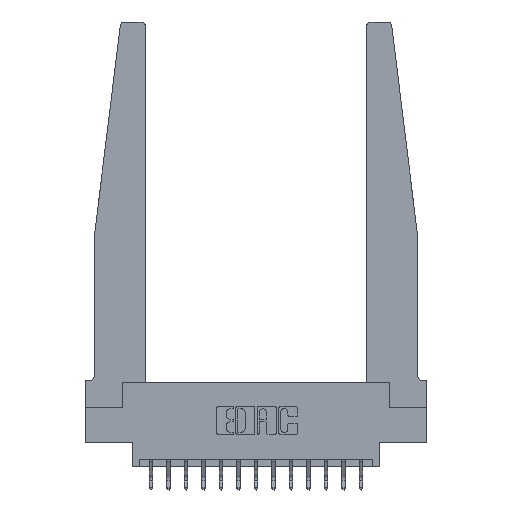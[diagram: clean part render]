
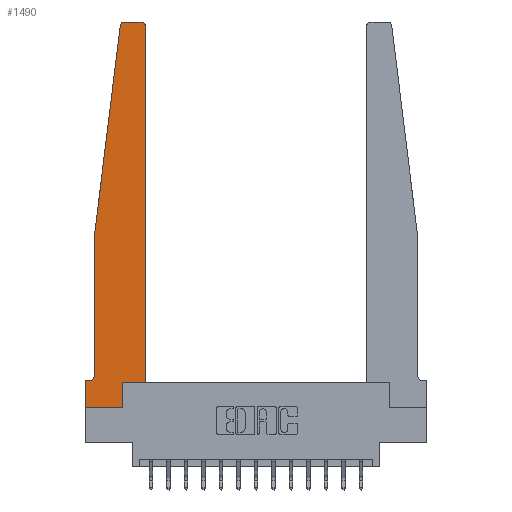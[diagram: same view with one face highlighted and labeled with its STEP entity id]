
A CAD part, top view. The second image highlights one B-rep face of the part: STEP entity #1490.
In plain terms, the highlighted planar face has unit normal (0, 0, 1).
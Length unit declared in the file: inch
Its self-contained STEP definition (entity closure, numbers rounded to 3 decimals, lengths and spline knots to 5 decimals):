
#187 = VECTOR ( 'NONE', #11471, 39.37008 ) ;
#728 = CARTESIAN_POINT ( 'NONE',  ( 0.25, 2.75, 0.37 ) ) ;
#776 = CARTESIAN_POINT ( 'NONE',  ( 0., 0., 0.37 ) ) ;
#872 = VERTEX_POINT ( 'NONE', #11358 ) ;
#966 = ORIENTED_EDGE ( 'NONE', *, *, #14735, .T. ) ;
#1274 = CARTESIAN_POINT ( 'NONE',  ( 0.065, 1.25, 0.37 ) ) ;
#1490 = ADVANCED_FACE ( 'NONE', ( #2339 ), #7859, .T. ) ;
#1570 = EDGE_CURVE ( 'NONE', #10822, #872, #14530, .T. ) ;
#1797 = DIRECTION ( 'NONE',  ( 0., 1., 0. ) ) ;
#1819 = CARTESIAN_POINT ( 'NONE',  ( 0.015, 0.1875, 0.37 ) ) ;
#1842 = CARTESIAN_POINT ( 'NONE',  ( 0.065, 1.25, 0.37 ) ) ;
#2105 = DIRECTION ( 'NONE',  ( -1., 0., 0. ) ) ;
#2115 = CARTESIAN_POINT ( 'NONE',  ( 0.065, 0.1875, 0.37 ) ) ;
#2339 = FACE_OUTER_BOUND ( 'NONE', #6630, .T. ) ;
#2379 = VERTEX_POINT ( 'NONE', #7065 ) ;
#2647 = AXIS2_PLACEMENT_3D ( 'NONE', #6317, #8947, #15874 ) ;
#2870 = CARTESIAN_POINT ( 'NONE',  ( 0., 0., 0.37 ) ) ;
#3141 = CARTESIAN_POINT ( 'NONE',  ( 0., 0., 0.37 ) ) ;
#3381 = LINE ( 'NONE', #2115, #16720 ) ;
#3712 = EDGE_CURVE ( 'NONE', #8958, #10822, #7441, .T. ) ;
#3829 = DIRECTION ( 'NONE',  ( -1., 0., 0. ) ) ;
#3869 = CARTESIAN_POINT ( 'NONE',  ( 0.395, 2.75, 0.37 ) ) ;
#3873 = CARTESIAN_POINT ( 'NONE',  ( 0.425, 0.18, 0.37 ) ) ;
#3912 = EDGE_CURVE ( 'NONE', #17514, #8958, #4047, .T. ) ;
#4047 = CIRCLE ( 'NONE', #14783, 0.03 ) ;
#4103 = CARTESIAN_POINT ( 'NONE',  ( 0.015, 0.2375, 0.37 ) ) ;
#4135 = DIRECTION ( 'NONE',  ( 1., 0., 0. ) ) ;
#4212 = LINE ( 'NONE', #2870, #187 ) ;
#4487 = DIRECTION ( 'NONE',  ( 0., 0., 1. ) ) ;
#4674 = EDGE_CURVE ( 'NONE', #11817, #5518, #9313, .T. ) ;
#4804 = DIRECTION ( 'NONE',  ( 0., -1., 0. ) ) ;
#4832 = ORIENTED_EDGE ( 'NONE', *, *, #9189, .T. ) ;
#4980 = EDGE_CURVE ( 'NONE', #16429, #11817, #14541, .T. ) ;
#5044 = ORIENTED_EDGE ( 'NONE', *, *, #12420, .T. ) ;
#5389 = CARTESIAN_POINT ( 'NONE',  ( 0.27653, 2.72, 0.37 ) ) ;
#5518 = VERTEX_POINT ( 'NONE', #1819 ) ;
#5753 = LINE ( 'NONE', #3141, #9712 ) ;
#5866 = EDGE_CURVE ( 'NONE', #2379, #6545, #16108, .T. ) ;
#5944 = CARTESIAN_POINT ( 'NONE',  ( 0.2605, 0.18, 0.37 ) ) ;
#6261 = DIRECTION ( 'NONE',  ( -0.122, -0.992, 0. ) ) ;
#6317 = CARTESIAN_POINT ( 'NONE',  ( 0., 0.1875, 0.37 ) ) ;
#6444 = CARTESIAN_POINT ( 'NONE',  ( 0.065, 0.2375, 0.37 ) ) ;
#6513 = ORIENTED_EDGE ( 'NONE', *, *, #3912, .T. ) ;
#6520 = VERTEX_POINT ( 'NONE', #12707 ) ;
#6545 = VERTEX_POINT ( 'NONE', #11354 ) ;
#6630 = EDGE_LOOP ( 'NONE', ( #7968, #7197, #15585, #8820, #7789, #17187, #966, #5044, #9394, #7447, #4832, #6513 ) ) ;
#6703 = VECTOR ( 'NONE', #7310, 39.37008 ) ;
#7065 = CARTESIAN_POINT ( 'NONE',  ( 0.2605, 0., 0.37 ) ) ;
#7138 = DIRECTION ( 'NONE',  ( 1., 0., 0. ) ) ;
#7197 = ORIENTED_EDGE ( 'NONE', *, *, #1570, .T. ) ;
#7273 = AXIS2_PLACEMENT_3D ( 'NONE', #5389, #8037, #4135 ) ;
#7310 = DIRECTION ( 'NONE',  ( 0., 1., 0. ) ) ;
#7441 = LINE ( 'NONE', #728, #13021 ) ;
#7447 = ORIENTED_EDGE ( 'NONE', *, *, #10141, .T. ) ;
#7627 = DIRECTION ( 'NONE',  ( -1., 0., 0. ) ) ;
#7662 = LINE ( 'NONE', #8931, #6703 ) ;
#7789 = ORIENTED_EDGE ( 'NONE', *, *, #4674, .T. ) ;
#7859 = PLANE ( 'NONE',  #2647 ) ;
#7914 = DIRECTION ( 'NONE',  ( 0., 0., -1. ) ) ;
#7968 = ORIENTED_EDGE ( 'NONE', *, *, #3712, .T. ) ;
#8037 = DIRECTION ( 'NONE',  ( 0., 0., 1. ) ) ;
#8201 = VECTOR ( 'NONE', #17510, 39.37008 ) ;
#8820 = ORIENTED_EDGE ( 'NONE', *, *, #4980, .T. ) ;
#8931 = CARTESIAN_POINT ( 'NONE',  ( 0.425, 0.18, 0.37 ) ) ;
#8947 = DIRECTION ( 'NONE',  ( 0., 0., 1. ) ) ;
#8958 = VERTEX_POINT ( 'NONE', #3869 ) ;
#8994 = CARTESIAN_POINT ( 'NONE',  ( 0.065, 1.25, 0.37 ) ) ;
#9000 = AXIS2_PLACEMENT_3D ( 'NONE', #4103, #7914, #3829 ) ;
#9189 = EDGE_CURVE ( 'NONE', #13513, #17514, #7662, .T. ) ;
#9313 = CIRCLE ( 'NONE', #9000, 0.05 ) ;
#9394 = ORIENTED_EDGE ( 'NONE', *, *, #5866, .T. ) ;
#9695 = CARTESIAN_POINT ( 'NONE',  ( 0.425, 2.72, 0.37 ) ) ;
#9712 = VECTOR ( 'NONE', #14116, 39.37008 ) ;
#10141 = EDGE_CURVE ( 'NONE', #6545, #13513, #14599, .T. ) ;
#10149 = CARTESIAN_POINT ( 'NONE',  ( 0.27653, 2.75, 0.37 ) ) ;
#10641 = VERTEX_POINT ( 'NONE', #776 ) ;
#10822 = VERTEX_POINT ( 'NONE', #10149 ) ;
#11354 = CARTESIAN_POINT ( 'NONE',  ( 0.2605, 0.18, 0.37 ) ) ;
#11358 = CARTESIAN_POINT ( 'NONE',  ( 0.24675, 2.72367, 0.37 ) ) ;
#11471 = DIRECTION ( 'NONE',  ( 0., -1., 0. ) ) ;
#11817 = VERTEX_POINT ( 'NONE', #6444 ) ;
#11955 = CARTESIAN_POINT ( 'NONE',  ( 0.425, 0.18, 0.37 ) ) ;
#12420 = EDGE_CURVE ( 'NONE', #10641, #2379, #5753, .T. ) ;
#12707 = CARTESIAN_POINT ( 'NONE',  ( 0., 0.1875, 0.37 ) ) ;
#13021 = VECTOR ( 'NONE', #2105, 39.37008 ) ;
#13271 = LINE ( 'NONE', #8994, #13532 ) ;
#13513 = VERTEX_POINT ( 'NONE', #3873 ) ;
#13532 = VECTOR ( 'NONE', #6261, 39.37008 ) ;
#14102 = EDGE_CURVE ( 'NONE', #5518, #6520, #3381, .T. ) ;
#14116 = DIRECTION ( 'NONE',  ( 1., 0., 0. ) ) ;
#14530 = CIRCLE ( 'NONE', #7273, 0.03 ) ;
#14541 = LINE ( 'NONE', #1842, #15602 ) ;
#14599 = LINE ( 'NONE', #11955, #8201 ) ;
#14735 = EDGE_CURVE ( 'NONE', #6520, #10641, #4212, .T. ) ;
#14783 = AXIS2_PLACEMENT_3D ( 'NONE', #15337, #4487, #7138 ) ;
#15227 = EDGE_CURVE ( 'NONE', #872, #16429, #13271, .T. ) ;
#15337 = CARTESIAN_POINT ( 'NONE',  ( 0.395, 2.72, 0.37 ) ) ;
#15585 = ORIENTED_EDGE ( 'NONE', *, *, #15227, .T. ) ;
#15602 = VECTOR ( 'NONE', #4804, 39.37008 ) ;
#15874 = DIRECTION ( 'NONE',  ( 1., 0., 0. ) ) ;
#16108 = LINE ( 'NONE', #5944, #17842 ) ;
#16429 = VERTEX_POINT ( 'NONE', #1274 ) ;
#16720 = VECTOR ( 'NONE', #7627, 39.37008 ) ;
#17187 = ORIENTED_EDGE ( 'NONE', *, *, #14102, .T. ) ;
#17510 = DIRECTION ( 'NONE',  ( 1., 0., 0. ) ) ;
#17514 = VERTEX_POINT ( 'NONE', #9695 ) ;
#17842 = VECTOR ( 'NONE', #1797, 39.37008 ) ;
